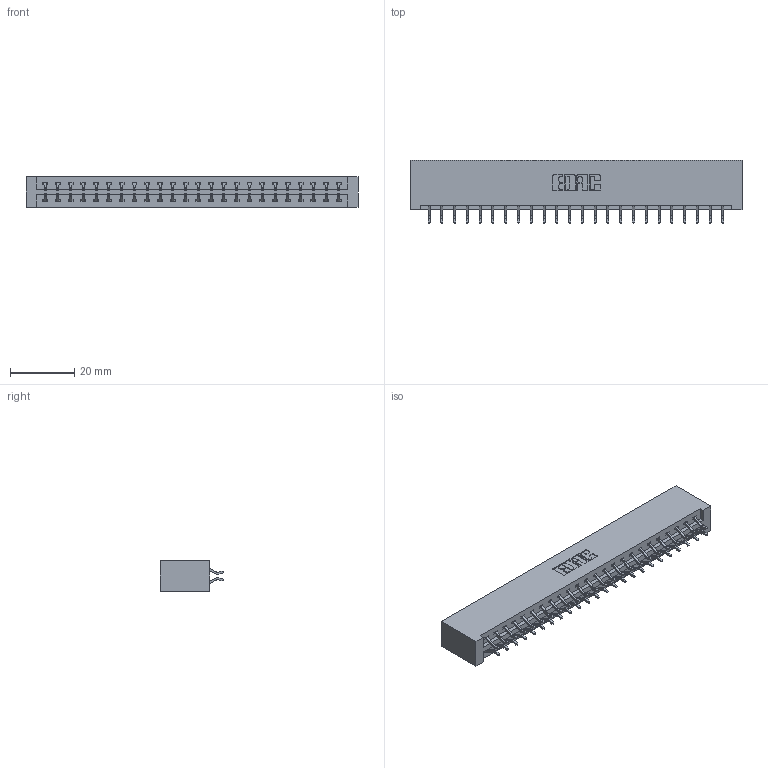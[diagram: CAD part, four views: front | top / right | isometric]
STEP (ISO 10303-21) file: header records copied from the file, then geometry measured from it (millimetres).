
FILE_DESCRIPTION (( 'STEP AP203' ), '1' );
FILE_NAME ('387-048-556-201.STEP', '2018-09-20T06:36:25', ( '' ), ( '' ), 'SwSTEP 2.0', 'SolidWorks 2016', '' );
FILE_SCHEMA (( 'CONFIG_CONTROL_DESIGN' ));
Length unit declared in the file: inch
Products named in the file (3): 387-048-556-201; 337 Part_No Mounting Lugs; 345-292-001_556 Tail
Assembly tree (49 placements, depth 2):
  387-048-556-201
    337 Part_No Mounting Lugs
    345-292-001_556 Tail  x48
Bounding box: 102.97 x 19.57 x 9.4 mm (x, y, z)
Volume: 11371.2 mm3; surface area: 12685.8 mm2
Topology: 49 solids, 49 shells, 2986 faces, 8879 edges, 5854 vertices
Faces by surface type: plane 2082, cylinder 904
Entity records: 20879 total; most frequent: CARTESIAN_POINT 3546, ORIENTED_EDGE 3470, DIRECTION 3031, EDGE_CURVE 1735, LINE 1607, VECTOR 1607, VERTEX_POINT 1154, AXIS2_PLACEMENT_3D 712
